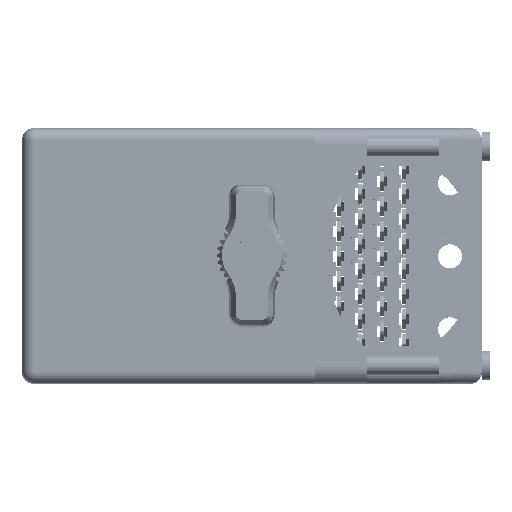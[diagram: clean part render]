
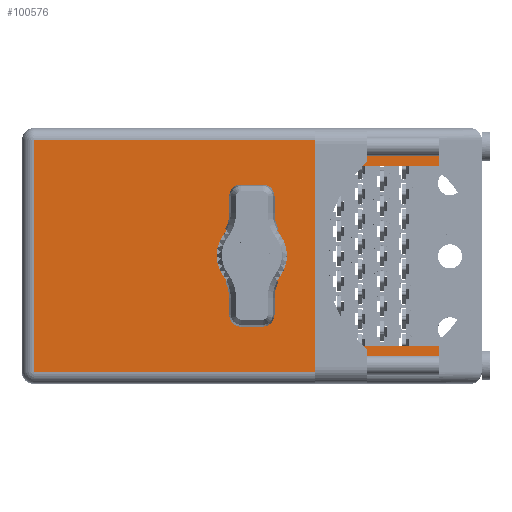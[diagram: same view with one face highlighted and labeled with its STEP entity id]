
A CAD part, top view. The second image highlights one B-rep face of the part: STEP entity #100576.
In plain terms, the highlighted face is planar.
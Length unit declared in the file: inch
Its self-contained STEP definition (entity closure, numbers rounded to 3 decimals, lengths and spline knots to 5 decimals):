
#72 = VECTOR ( 'NONE', #75708, 39.37008 ) ;
#764 = PLANE ( 'NONE',  #53881 ) ;
#1080 = CARTESIAN_POINT ( 'NONE',  ( 0.07, 2.03, -1.46 ) ) ;
#1620 = CARTESIAN_POINT ( 'NONE',  ( 1.785, 2.03, -1.305 ) ) ;
#2008 = CARTESIAN_POINT ( 'NONE',  ( 2.499, 2.03, -0.225 ) ) ;
#2866 = ORIENTED_EDGE ( 'NONE', *, *, #92746, .F. ) ;
#2875 = DIRECTION ( 'NONE',  ( 1., 0., 0. ) ) ;
#3845 = DIRECTION ( 'NONE',  ( 0., 0., 1. ) ) ;
#4215 = DIRECTION ( 'NONE',  ( 0., 1., 0. ) ) ;
#8202 = FACE_OUTER_BOUND ( 'NONE', #8442, .T. ) ;
#8404 = LINE ( 'NONE', #65828, #13733 ) ;
#8442 = EDGE_LOOP ( 'NONE', ( #9182, #38185, #34900, #85525, #40784, #31153, #104407, #100372 ) ) ;
#9182 = ORIENTED_EDGE ( 'NONE', *, *, #38979, .T. ) ;
#9662 = EDGE_CURVE ( 'NONE', #17119, #69833, #17966, .T. ) ;
#12329 = CARTESIAN_POINT ( 'NONE',  ( 1.3775, 2.03, -0.765 ) ) ;
#13733 = VECTOR ( 'NONE', #83922, 39.37008 ) ;
#14051 = CARTESIAN_POINT ( 'NONE',  ( 1.785, 2.03, -0.225 ) ) ;
#14409 = VECTOR ( 'NONE', #49546, 39.37008 ) ;
#16426 = EDGE_CURVE ( 'NONE', #65987, #17119, #8404, .T. ) ;
#17061 = LINE ( 'NONE', #32996, #14409 ) ;
#17119 = VERTEX_POINT ( 'NONE', #14051 ) ;
#17966 = LINE ( 'NONE', #23795, #82712 ) ;
#21308 = CARTESIAN_POINT ( 'NONE',  ( 0., 2.03, -1.46 ) ) ;
#23795 = CARTESIAN_POINT ( 'NONE',  ( 1.785, 2.03, -1.305 ) ) ;
#31153 = ORIENTED_EDGE ( 'NONE', *, *, #58401, .T. ) ;
#31520 = EDGE_CURVE ( 'NONE', #65987, #105721, #37078, .T. ) ;
#32996 = CARTESIAN_POINT ( 'NONE',  ( 0.07, 2.03, -1.53 ) ) ;
#33662 = DIRECTION ( 'NONE',  ( 0., 1., 0. ) ) ;
#34900 = ORIENTED_EDGE ( 'NONE', *, *, #31520, .F. ) ;
#35518 = CARTESIAN_POINT ( 'NONE',  ( 1.3775, 2.03, -0.765 ) ) ;
#36386 = CARTESIAN_POINT ( 'NONE',  ( 2.499, 2.03, -1.46 ) ) ;
#37041 = CARTESIAN_POINT ( 'NONE',  ( 2.499, 2.03, -1.305 ) ) ;
#37078 = LINE ( 'NONE', #67177, #72 ) ;
#38185 = ORIENTED_EDGE ( 'NONE', *, *, #80741, .T. ) ;
#38639 = DIRECTION ( 'NONE',  ( -1., 0., 0. ) ) ;
#38979 = EDGE_CURVE ( 'NONE', #105208, #61643, #17061, .T. ) ;
#39916 = FACE_BOUND ( 'NONE', #66516, .T. ) ;
#40784 = ORIENTED_EDGE ( 'NONE', *, *, #9662, .T. ) ;
#41113 = CARTESIAN_POINT ( 'NONE',  ( 2.499, 2.03, -1.53 ) ) ;
#41502 = DIRECTION ( 'NONE',  ( 1., 0., 0. ) ) ;
#45268 = VECTOR ( 'NONE', #92377, 39.37008 ) ;
#49092 = VERTEX_POINT ( 'NONE', #70920 ) ;
#49546 = DIRECTION ( 'NONE',  ( 0., 0., 1. ) ) ;
#49942 = CARTESIAN_POINT ( 'NONE',  ( 0.07, 2.03, -0.07 ) ) ;
#50911 = VERTEX_POINT ( 'NONE', #36386 ) ;
#53881 = AXIS2_PLACEMENT_3D ( 'NONE', #84192, #33662, #101154 ) ;
#56317 = CARTESIAN_POINT ( 'NONE',  ( 2.499, 2.03, -1.305 ) ) ;
#58401 = EDGE_CURVE ( 'NONE', #69833, #108791, #104071, .T. ) ;
#61643 = VERTEX_POINT ( 'NONE', #49942 ) ;
#62292 = CARTESIAN_POINT ( 'NONE',  ( 2.499, 2.03, -0.07 ) ) ;
#63108 = VECTOR ( 'NONE', #41502, 39.37008 ) ;
#64671 = CARTESIAN_POINT ( 'NONE',  ( 1.3775, 2.03, -0.935 ) ) ;
#65828 = CARTESIAN_POINT ( 'NONE',  ( 2.499, 2.03, -0.225 ) ) ;
#65987 = VERTEX_POINT ( 'NONE', #2008 ) ;
#66516 = EDGE_LOOP ( 'NONE', ( #87615, #2866 ) ) ;
#67177 = CARTESIAN_POINT ( 'NONE',  ( 2.499, 2.03, -1.53 ) ) ;
#69833 = VERTEX_POINT ( 'NONE', #1620 ) ;
#70906 = CIRCLE ( 'NONE', #109256, 0.17 ) ;
#70920 = CARTESIAN_POINT ( 'NONE',  ( 1.3775, 2.03, -0.595 ) ) ;
#71375 = VERTEX_POINT ( 'NONE', #64671 ) ;
#72392 = LINE ( 'NONE', #62292, #77695 ) ;
#74731 = DIRECTION ( 'NONE',  ( 0., 0., -1. ) ) ;
#74966 = LINE ( 'NONE', #21308, #94723 ) ;
#75013 = EDGE_CURVE ( 'NONE', #50911, #105208, #74966, .T. ) ;
#75708 = DIRECTION ( 'NONE',  ( 0., 0., 1. ) ) ;
#77695 = VECTOR ( 'NONE', #2875, 39.37008 ) ;
#78618 = AXIS2_PLACEMENT_3D ( 'NONE', #35518, #93067, #94517 ) ;
#79143 = EDGE_CURVE ( 'NONE', #50911, #108791, #94073, .T. ) ;
#80741 = EDGE_CURVE ( 'NONE', #61643, #105721, #72392, .T. ) ;
#82712 = VECTOR ( 'NONE', #74731, 39.37008 ) ;
#83922 = DIRECTION ( 'NONE',  ( -1., 0., 0. ) ) ;
#84192 = CARTESIAN_POINT ( 'NONE',  ( 0., 2.03, -1.53 ) ) ;
#85525 = ORIENTED_EDGE ( 'NONE', *, *, #16426, .T. ) ;
#87615 = ORIENTED_EDGE ( 'NONE', *, *, #88861, .F. ) ;
#88857 = CIRCLE ( 'NONE', #78618, 0.17 ) ;
#88861 = EDGE_CURVE ( 'NONE', #49092, #71375, #88857, .T. ) ;
#92377 = DIRECTION ( 'NONE',  ( 0., 0., 1. ) ) ;
#92746 = EDGE_CURVE ( 'NONE', #71375, #49092, #70906, .T. ) ;
#93067 = DIRECTION ( 'NONE',  ( 0., 1., 0. ) ) ;
#94073 = LINE ( 'NONE', #41113, #45268 ) ;
#94517 = DIRECTION ( 'NONE',  ( 0., 0., 1. ) ) ;
#94723 = VECTOR ( 'NONE', #38639, 39.37008 ) ;
#98827 = CARTESIAN_POINT ( 'NONE',  ( 2.499, 2.03, -0.07 ) ) ;
#100372 = ORIENTED_EDGE ( 'NONE', *, *, #75013, .T. ) ;
#100576 = ADVANCED_FACE ( 'NONE', ( #8202, #39916 ), #764, .T. ) ;
#101154 = DIRECTION ( 'NONE',  ( 0., 0., 1. ) ) ;
#104071 = LINE ( 'NONE', #56317, #63108 ) ;
#104407 = ORIENTED_EDGE ( 'NONE', *, *, #79143, .F. ) ;
#105208 = VERTEX_POINT ( 'NONE', #1080 ) ;
#105721 = VERTEX_POINT ( 'NONE', #98827 ) ;
#108791 = VERTEX_POINT ( 'NONE', #37041 ) ;
#109256 = AXIS2_PLACEMENT_3D ( 'NONE', #12329, #4215, #3845 ) ;
